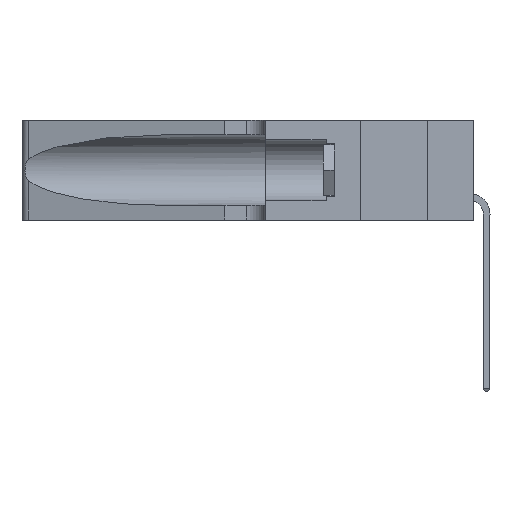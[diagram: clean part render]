
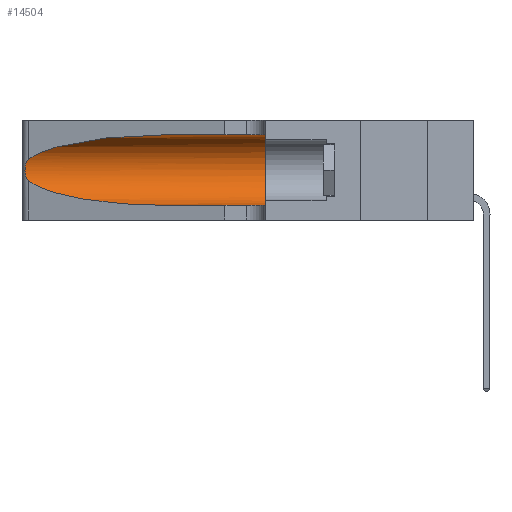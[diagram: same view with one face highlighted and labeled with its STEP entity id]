
A CAD part, left-side view. The second image highlights one B-rep face of the part: STEP entity #14504.
In plain terms, the highlighted cylindrical face has radius 3.308 mm (diameter 6.617 mm), a partial arc.
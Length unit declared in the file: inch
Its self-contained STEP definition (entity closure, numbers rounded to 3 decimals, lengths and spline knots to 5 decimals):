
#504 = CARTESIAN_POINT ( 'NONE',  ( 0.25487, 1.22718, 0.14631 ) ) ;
#1087 = ORIENTED_EDGE ( 'NONE', *, *, #13018, .T. ) ;
#1663 = LINE ( 'NONE', #8491, #5156 ) ;
#1713 = ORIENTED_EDGE ( 'NONE', *, *, #21152, .F. ) ;
#2390 = VERTEX_POINT ( 'NONE', #2640 ) ;
#2518 = CARTESIAN_POINT ( 'NONE',  ( 0.26075, 1.23896, 0.178 ) ) ;
#2640 = CARTESIAN_POINT ( 'NONE',  ( 0.1305, 0.35, 0.05475 ) ) ;
#3996 = DIRECTION ( 'NONE',  ( 0., -1., 0. ) ) ;
#4456 = ORIENTED_EDGE ( 'NONE', *, *, #28153, .T. ) ;
#4816 = CARTESIAN_POINT ( 'NONE',  ( 0.1305, 0.72297, 0.31525 ) ) ;
#5156 = VECTOR ( 'NONE', #31270, 39.37008 ) ;
#5226 = AXIS2_PLACEMENT_3D ( 'NONE', #20212, #10224, #5317 ) ;
#5317 = DIRECTION ( 'NONE',  ( 0., 0., 1. ) ) ;
#5488 = AXIS2_PLACEMENT_3D ( 'NONE', #13906, #3996, #28776 ) ;
#5580 = CARTESIAN_POINT ( 'NONE',  ( 0.1305, 1.61858, 0.31525 ) ) ;
#8491 = CARTESIAN_POINT ( 'NONE',  ( 0.1305, 1.61858, 0.05475 ) ) ;
#9131 = EDGE_CURVE ( 'NONE', #21048, #18130, #31550, .T. ) ;
#10224 = DIRECTION ( 'NONE',  ( 0., 1., 0. ) ) ;
#11067 = CARTESIAN_POINT ( 'NONE',  ( 0.25787, 1.23484, 0.2124 ) ) ;
#11302 =( BOUNDED_CURVE ( )  B_SPLINE_CURVE ( 3, ( #15384, #20778, #30392, #30594 ),
 .UNSPECIFIED., .F., .F. ) 
 B_SPLINE_CURVE_WITH_KNOTS ( ( 4, 4 ),
 ( 3.44316, 4.71239 ),
 .UNSPECIFIED. ) 
 CURVE ( )  GEOMETRIC_REPRESENTATION_ITEM ( )  RATIONAL_B_SPLINE_CURVE ( ( 1., 0.87, 0.87, 1. ) ) 
 REPRESENTATION_ITEM ( '' )  );
#13018 = EDGE_CURVE ( 'NONE', #31538, #2390, #1663, .T. ) ;
#13428 = CARTESIAN_POINT ( 'NONE',  ( 0.26018, 1.23835, 0.19895 ) ) ;
#13460 = CYLINDRICAL_SURFACE ( 'NONE', #5488, 0.13025 ) ;
#13810 = CARTESIAN_POINT ( 'NONE',  ( 0.1305, 0.35, 0.31525 ) ) ;
#13906 = CARTESIAN_POINT ( 'NONE',  ( 0.1305, 1.61858, 0.185 ) ) ;
#14504 = ADVANCED_FACE ( 'NONE', ( #32371 ), #13460, .F. ) ;
#15190 = CARTESIAN_POINT ( 'NONE',  ( 0.26075, 1.23896, 0.19203 ) ) ;
#15384 = CARTESIAN_POINT ( 'NONE',  ( 0.25487, 1.22718, 0.14631 ) ) ;
#15736 = CARTESIAN_POINT ( 'NONE',  ( 0.25555, 1.22993, 0.14849 ) ) ;
#15972 = CARTESIAN_POINT ( 'NONE',  ( 0.25789, 1.23486, 0.15765 ) ) ;
#16097 = CARTESIAN_POINT ( 'NONE',  ( 0.25555, 1.22994, 0.2215 ) ) ;
#17515 = LINE ( 'NONE', #5580, #19485 ) ;
#18089 = EDGE_LOOP ( 'NONE', ( #20883, #4456, #19991, #1087, #1713, #21558 ) ) ;
#18130 = VERTEX_POINT ( 'NONE', #19103 ) ;
#18756 = DIRECTION ( 'NONE',  ( 0., -1., 0. ) ) ;
#19103 = CARTESIAN_POINT ( 'NONE',  ( 0.25487, 1.22718, 0.22369 ) ) ;
#19485 = VECTOR ( 'NONE', #18756, 39.37008 ) ;
#19991 = ORIENTED_EDGE ( 'NONE', *, *, #24165, .T. ) ;
#20212 = CARTESIAN_POINT ( 'NONE',  ( 0.1305, 0.35, 0.185 ) ) ;
#20778 = CARTESIAN_POINT ( 'NONE',  ( 0.2373, 1.15595, 0.08982 ) ) ;
#20883 = ORIENTED_EDGE ( 'NONE', *, *, #9131, .T. ) ;
#21048 = VERTEX_POINT ( 'NONE', #4816 ) ;
#21152 = EDGE_CURVE ( 'NONE', #22818, #2390, #23180, .T. ) ;
#21232 = CARTESIAN_POINT ( 'NONE',  ( 0.25487, 1.22718, 0.22369 ) ) ;
#21558 = ORIENTED_EDGE ( 'NONE', *, *, #28173, .F. ) ;
#21666 = B_SPLINE_CURVE_WITH_KNOTS ( 'NONE', 3,
 ( #25983, #16097, #26230, #11067, #28775, #13428, #15190, #2518, #22810, #28297, #15972, #30822, #15736, #504 ),
 .UNSPECIFIED., .F., .F.,
 ( 4, 2, 2, 2, 2, 2, 4 ),
 ( 0., 0.00027, 0.00053, 0.00107, 0.0016, 0.00187, 0.00214 ),
 .UNSPECIFIED. ) ;
#22649 = CARTESIAN_POINT ( 'NONE',  ( 0.1305, 0.72297, 0.05475 ) ) ;
#22810 = CARTESIAN_POINT ( 'NONE',  ( 0.26017, 1.23833, 0.17102 ) ) ;
#22818 = VERTEX_POINT ( 'NONE', #13810 ) ;
#23180 = CIRCLE ( 'NONE', #5226, 0.13025 ) ;
#23297 = CARTESIAN_POINT ( 'NONE',  ( 0.18966, 0.96281, 0.31525 ) ) ;
#23641 = CARTESIAN_POINT ( 'NONE',  ( 0.1305, 0.72297, 0.31525 ) ) ;
#24165 = EDGE_CURVE ( 'NONE', #31033, #31538, #11302, .T. ) ;
#25934 = CARTESIAN_POINT ( 'NONE',  ( 0.2373, 1.15595, 0.28018 ) ) ;
#25983 = CARTESIAN_POINT ( 'NONE',  ( 0.25487, 1.22718, 0.22369 ) ) ;
#26230 = CARTESIAN_POINT ( 'NONE',  ( 0.25639, 1.23184, 0.21858 ) ) ;
#28153 = EDGE_CURVE ( 'NONE', #18130, #31033, #21666, .T. ) ;
#28173 = EDGE_CURVE ( 'NONE', #21048, #22818, #17515, .T. ) ;
#28297 = CARTESIAN_POINT ( 'NONE',  ( 0.25856, 1.23593, 0.16098 ) ) ;
#28775 = CARTESIAN_POINT ( 'NONE',  ( 0.25854, 1.2359, 0.20912 ) ) ;
#28776 = DIRECTION ( 'NONE',  ( 0., 0., -1. ) ) ;
#30392 = CARTESIAN_POINT ( 'NONE',  ( 0.18966, 0.96281, 0.05475 ) ) ;
#30594 = CARTESIAN_POINT ( 'NONE',  ( 0.1305, 0.72297, 0.05475 ) ) ;
#30822 = CARTESIAN_POINT ( 'NONE',  ( 0.25639, 1.23186, 0.15144 ) ) ;
#31033 = VERTEX_POINT ( 'NONE', #32671 ) ;
#31270 = DIRECTION ( 'NONE',  ( 0., -1., 0. ) ) ;
#31538 = VERTEX_POINT ( 'NONE', #22649 ) ;
#31550 =( BOUNDED_CURVE ( )  B_SPLINE_CURVE ( 3, ( #23641, #23297, #25934, #21232 ),
 .UNSPECIFIED., .F., .F. ) 
 B_SPLINE_CURVE_WITH_KNOTS ( ( 4, 4 ),
 ( 1.5708, 2.84003 ),
 .UNSPECIFIED. ) 
 CURVE ( )  GEOMETRIC_REPRESENTATION_ITEM ( )  RATIONAL_B_SPLINE_CURVE ( ( 1., 0.87, 0.87, 1. ) ) 
 REPRESENTATION_ITEM ( '' )  );
#32371 = FACE_OUTER_BOUND ( 'NONE', #18089, .T. ) ;
#32671 = CARTESIAN_POINT ( 'NONE',  ( 0.25487, 1.22718, 0.14631 ) ) ;
